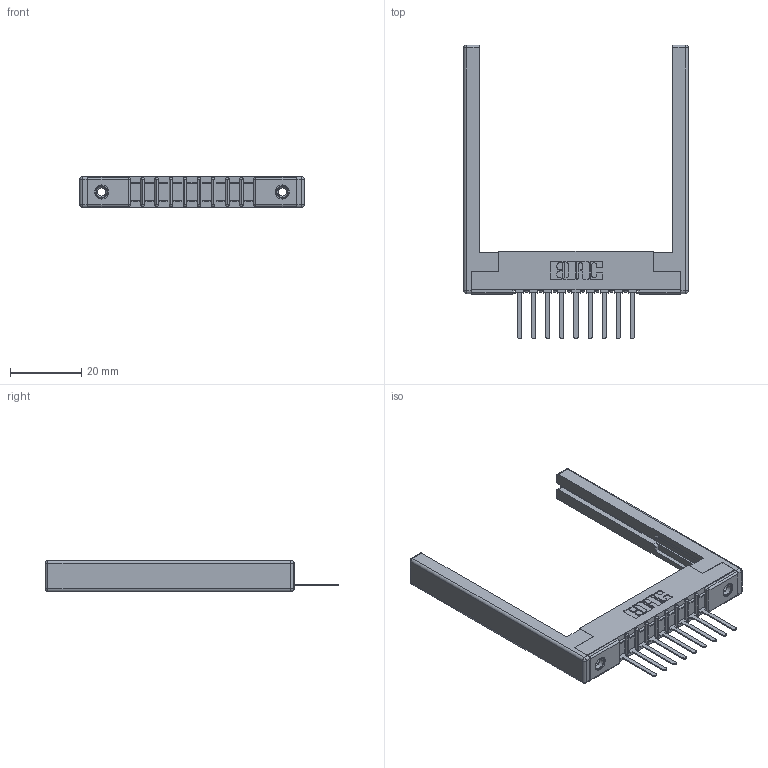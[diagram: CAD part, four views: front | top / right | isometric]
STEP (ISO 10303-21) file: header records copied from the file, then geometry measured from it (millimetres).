
FILE_DESCRIPTION (( 'STEP AP203' ), '1' );
FILE_NAME ('307-009-441-168.STEP', '2020-09-25T06:10:18', ( '' ), ( '' ), 'SwSTEP 2.0', 'SolidWorks 2020', '' );
FILE_SCHEMA (( 'CONFIG_CONTROL_DESIGN' ));
Length unit declared in the file: inch
Products named in the file (5): 307-290-002_541; 345-250-001_345-250-001-102; 307 Part_.156 Dia Mounting Holes; 307-220-068; 307-009-441-168
Assembly tree (14 placements, depth 2):
  307-009-441-168
    307 Part_.156 Dia Mounting Holes
    307-290-002_541  x9
    307-220-068  x2
    345-250-001_345-250-001-102  x2
Bounding box: 63.09 x 82.55 x 8.71 mm (x, y, z)
Volume: 8742.7 mm3; surface area: 11060.9 mm2
Topology: 14 solids, 14 shells, 948 faces, 2801 edges, 1818 vertices
Faces by surface type: plane 563, cylinder 341, sphere 28, cone 12, torus 4
Entity records: 15261 total; most frequent: CARTESIAN_POINT 2533, ORIENTED_EDGE 2512, DIRECTION 2494, EDGE_CURVE 1256, LINE 944, VECTOR 944, VERTEX_POINT 814, AXIS2_PLACEMENT_3D 775
